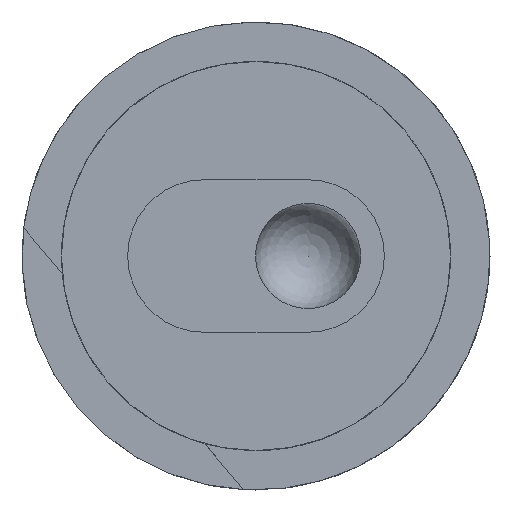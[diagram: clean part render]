
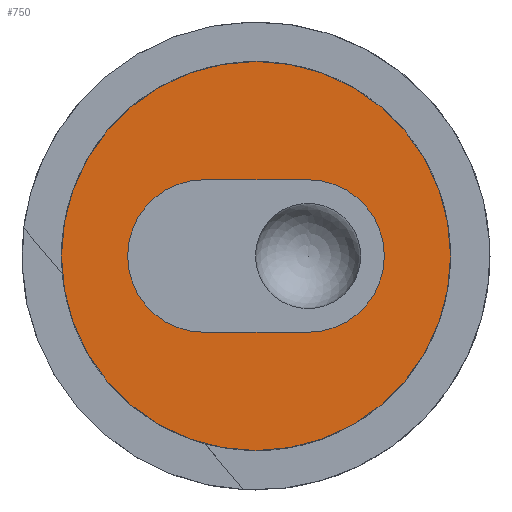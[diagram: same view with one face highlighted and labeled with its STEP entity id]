
A CAD part, front view. The second image highlights one B-rep face of the part: STEP entity #750.
In plain terms, the highlighted planar face has unit normal (0, -1, 0).
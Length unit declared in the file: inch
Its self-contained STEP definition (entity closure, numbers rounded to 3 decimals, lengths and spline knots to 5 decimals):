
#17=FACE_BOUND('',#129,.T.);
#37=PLANE('',#846);
#87=FACE_OUTER_BOUND('',#128,.T.);
#128=EDGE_LOOP('',(#695));
#129=EDGE_LOOP('',(#696,#697,#698,#699));
#143=CIRCLE('',#787,0.185);
#161=CIRCLE('',#817,0.0725);
#172=CIRCLE('',#840,0.0725);
#227=LINE('',#1359,#272);
#234=LINE('',#1398,#279);
#272=VECTOR('',#975,0.3937);
#279=VECTOR('',#1000,0.3937);
#312=VERTEX_POINT('',#1232);
#344=VERTEX_POINT('',#1356);
#345=VERTEX_POINT('',#1358);
#350=VERTEX_POINT('',#1376);
#354=VERTEX_POINT('',#1396);
#396=EDGE_CURVE('',#312,#312,#143,.F.);
#443=EDGE_CURVE('',#345,#344,#227,.F.);
#450=EDGE_CURVE('',#350,#344,#161,.T.);
#458=EDGE_CURVE('',#350,#354,#234,.F.);
#472=EDGE_CURVE('',#345,#354,#172,.T.);
#695=ORIENTED_EDGE('',*,*,#396,.T.);
#696=ORIENTED_EDGE('',*,*,#458,.T.);
#697=ORIENTED_EDGE('',*,*,#472,.F.);
#698=ORIENTED_EDGE('',*,*,#443,.T.);
#699=ORIENTED_EDGE('',*,*,#450,.F.);
#750=ADVANCED_FACE('',(#87,#17),#37,.F.);
#787=AXIS2_PLACEMENT_3D('',#1233,#898,#899);
#817=AXIS2_PLACEMENT_3D('',#1378,#983,#984);
#840=AXIS2_PLACEMENT_3D('',#1429,#1039,#1040);
#846=AXIS2_PLACEMENT_3D('',#1442,#1055,#1056);
#898=DIRECTION('center_axis',(0.,1.,0.));
#899=DIRECTION('ref_axis',(0.766,0.,0.643));
#975=DIRECTION('',(-1.,0.,0.));
#983=DIRECTION('center_axis',(0.,-1.,0.));
#984=DIRECTION('ref_axis',(0.707,0.,0.707));
#1000=DIRECTION('',(1.,0.,0.));
#1039=DIRECTION('center_axis',(0.,-1.,0.));
#1040=DIRECTION('ref_axis',(-0.707,0.,-0.707));
#1055=DIRECTION('center_axis',(0.,1.,0.));
#1056=DIRECTION('ref_axis',(0.766,0.,0.643));
#1232=CARTESIAN_POINT('',(-0.14172,-0.5975,0.10858));
#1233=CARTESIAN_POINT('Origin',(0.,-0.5975,0.2275));
#1356=CARTESIAN_POINT('',(0.0495,-0.5975,0.3));
#1358=CARTESIAN_POINT('',(-0.0495,-0.5975,0.3));
#1359=CARTESIAN_POINT('',(0.05,-0.5975,0.3));
#1376=CARTESIAN_POINT('',(0.0495,-0.5975,0.155));
#1378=CARTESIAN_POINT('Origin',(0.0495,-0.5975,0.2275));
#1396=CARTESIAN_POINT('',(-0.0495,-0.5975,0.155));
#1398=CARTESIAN_POINT('',(-0.05,-0.5975,0.155));
#1429=CARTESIAN_POINT('Origin',(-0.0495,-0.5975,0.2275));
#1442=CARTESIAN_POINT('Origin',(0.,-0.5975,0.2275));
